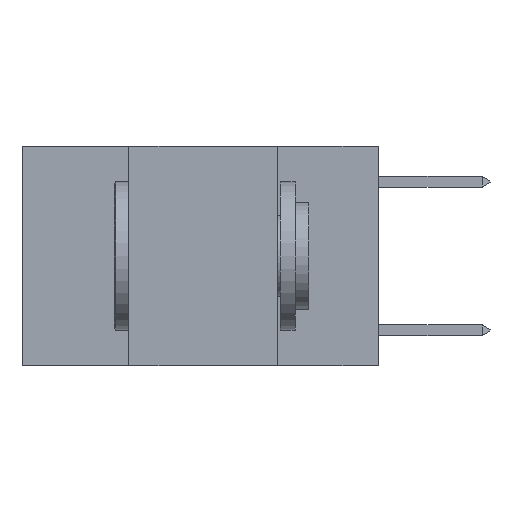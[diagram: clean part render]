
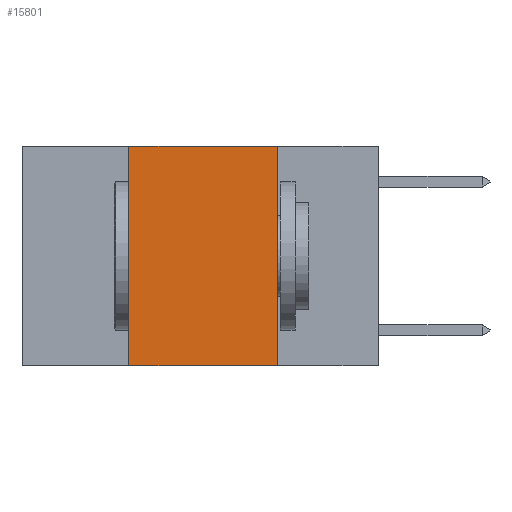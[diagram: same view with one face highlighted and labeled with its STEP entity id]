
A CAD part, left-side view. The second image highlights one B-rep face of the part: STEP entity #15801.
In plain terms, the highlighted planar face has unit normal (-1, 0, 0).
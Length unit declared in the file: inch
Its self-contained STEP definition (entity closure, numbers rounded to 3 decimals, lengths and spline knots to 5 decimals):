
#42 = VECTOR ( 'NONE', #2921, 39.37008 ) ;
#50 = DIRECTION ( 'NONE',  ( 0., -1., 0. ) ) ;
#839 = VERTEX_POINT ( 'NONE', #13490 ) ;
#1065 = LINE ( 'NONE', #3820, #10308 ) ;
#1500 = LINE ( 'NONE', #6726, #15774 ) ;
#1960 = ORIENTED_EDGE ( 'NONE', *, *, #11233, .T. ) ;
#2101 = CARTESIAN_POINT ( 'NONE',  ( 0., 0.17, -0.37 ) ) ;
#2658 = LINE ( 'NONE', #11781, #8471 ) ;
#2921 = DIRECTION ( 'NONE',  ( 0., 0., 1. ) ) ;
#3143 = VERTEX_POINT ( 'NONE', #15617 ) ;
#3820 = CARTESIAN_POINT ( 'NONE',  ( 0., 0.6, -0.37 ) ) ;
#4110 = LINE ( 'NONE', #7084, #42 ) ;
#4512 = ORIENTED_EDGE ( 'NONE', *, *, #6598, .F. ) ;
#4534 = ORIENTED_EDGE ( 'NONE', *, *, #10435, .F. ) ;
#5262 = FACE_OUTER_BOUND ( 'NONE', #8020, .T. ) ;
#5281 = CARTESIAN_POINT ( 'NONE',  ( 0., 0.42, -0.37 ) ) ;
#6186 = DIRECTION ( 'NONE',  ( 0., -1., 0. ) ) ;
#6390 = CARTESIAN_POINT ( 'NONE',  ( 0., 0.6, 0. ) ) ;
#6598 = EDGE_CURVE ( 'NONE', #839, #9615, #2658, .T. ) ;
#6726 = CARTESIAN_POINT ( 'NONE',  ( 0., 0.6, 0. ) ) ;
#7084 = CARTESIAN_POINT ( 'NONE',  ( 0., 0.42, 0. ) ) ;
#8020 = EDGE_LOOP ( 'NONE', ( #4512, #12223, #4534, #1960 ) ) ;
#8471 = VECTOR ( 'NONE', #13059, 39.37008 ) ;
#9615 = VERTEX_POINT ( 'NONE', #2101 ) ;
#10282 = AXIS2_PLACEMENT_3D ( 'NONE', #6390, #15814, #10468 ) ;
#10308 = VECTOR ( 'NONE', #6186, 39.37008 ) ;
#10435 = EDGE_CURVE ( 'NONE', #15077, #3143, #4110, .T. ) ;
#10468 = DIRECTION ( 'NONE',  ( 0., 0., -1. ) ) ;
#10654 = PLANE ( 'NONE',  #10282 ) ;
#11233 = EDGE_CURVE ( 'NONE', #15077, #9615, #1065, .T. ) ;
#11781 = CARTESIAN_POINT ( 'NONE',  ( 0., 0.17, 0. ) ) ;
#12223 = ORIENTED_EDGE ( 'NONE', *, *, #14245, .F. ) ;
#13059 = DIRECTION ( 'NONE',  ( 0., 0., -1. ) ) ;
#13490 = CARTESIAN_POINT ( 'NONE',  ( 0., 0.17, 0. ) ) ;
#14245 = EDGE_CURVE ( 'NONE', #3143, #839, #1500, .T. ) ;
#15077 = VERTEX_POINT ( 'NONE', #5281 ) ;
#15617 = CARTESIAN_POINT ( 'NONE',  ( 0., 0.42, 0. ) ) ;
#15774 = VECTOR ( 'NONE', #50, 39.37008 ) ;
#15801 = ADVANCED_FACE ( 'NONE', ( #5262 ), #10654, .F. ) ;
#15814 = DIRECTION ( 'NONE',  ( 1., 0., 0. ) ) ;
